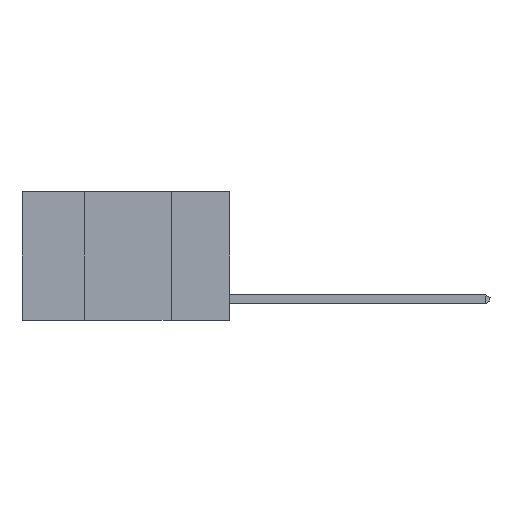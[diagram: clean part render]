
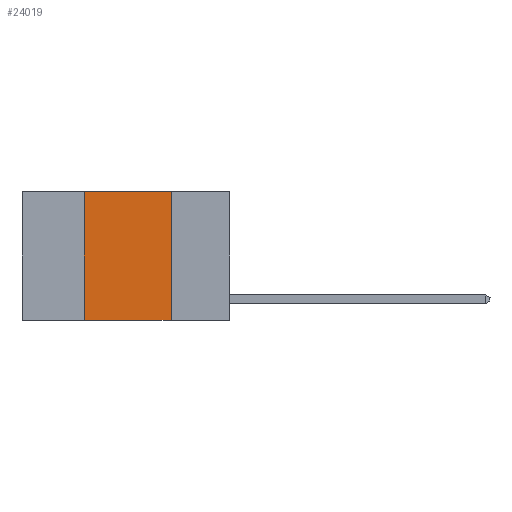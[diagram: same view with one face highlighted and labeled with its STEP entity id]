
A CAD part, left-side view. The second image highlights one B-rep face of the part: STEP entity #24019.
In plain terms, the highlighted planar face has unit normal (-1, 0, 0).
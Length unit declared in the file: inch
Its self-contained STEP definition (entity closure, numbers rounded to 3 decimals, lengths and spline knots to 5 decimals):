
#292 = LINE ( 'NONE', #28419, #7447 ) ;
#491 = CARTESIAN_POINT ( 'NONE',  ( 0., 0.17, 0. ) ) ;
#982 = EDGE_LOOP ( 'NONE', ( #23580, #26394, #14096, #22156 ) ) ;
#1614 = VECTOR ( 'NONE', #18758, 39.37008 ) ;
#3775 = EDGE_CURVE ( 'NONE', #6703, #23410, #18141, .T. ) ;
#4609 = CARTESIAN_POINT ( 'NONE',  ( 0., 0.6, -0.37 ) ) ;
#5477 = DIRECTION ( 'NONE',  ( 0., 0., -1. ) ) ;
#5719 = DIRECTION ( 'NONE',  ( 0., 0., -1. ) ) ;
#6703 = VERTEX_POINT ( 'NONE', #7699 ) ;
#6987 = DIRECTION ( 'NONE',  ( 0., 0., 1. ) ) ;
#7192 = LINE ( 'NONE', #4609, #1614 ) ;
#7447 = VECTOR ( 'NONE', #6987, 39.37008 ) ;
#7699 = CARTESIAN_POINT ( 'NONE',  ( 0., 0.42, 0. ) ) ;
#8982 = VECTOR ( 'NONE', #5719, 39.37008 ) ;
#11520 = VERTEX_POINT ( 'NONE', #12264 ) ;
#12264 = CARTESIAN_POINT ( 'NONE',  ( 0., 0.17, -0.37 ) ) ;
#12761 = CARTESIAN_POINT ( 'NONE',  ( 0., 0.6, 0. ) ) ;
#13286 = DIRECTION ( 'NONE',  ( 0., -1., 0. ) ) ;
#14096 = ORIENTED_EDGE ( 'NONE', *, *, #27547, .F. ) ;
#15358 = EDGE_CURVE ( 'NONE', #17722, #11520, #7192, .T. ) ;
#17275 = LINE ( 'NONE', #23964, #8982 ) ;
#17393 = VECTOR ( 'NONE', #13286, 39.37008 ) ;
#17722 = VERTEX_POINT ( 'NONE', #18951 ) ;
#18141 = LINE ( 'NONE', #29403, #17393 ) ;
#18758 = DIRECTION ( 'NONE',  ( 0., -1., 0. ) ) ;
#18951 = CARTESIAN_POINT ( 'NONE',  ( 0., 0.42, -0.37 ) ) ;
#19206 = EDGE_CURVE ( 'NONE', #23410, #11520, #17275, .T. ) ;
#22071 = DIRECTION ( 'NONE',  ( 1., 0., 0. ) ) ;
#22156 = ORIENTED_EDGE ( 'NONE', *, *, #15358, .T. ) ;
#23241 = AXIS2_PLACEMENT_3D ( 'NONE', #12761, #22071, #5477 ) ;
#23410 = VERTEX_POINT ( 'NONE', #491 ) ;
#23580 = ORIENTED_EDGE ( 'NONE', *, *, #19206, .F. ) ;
#23964 = CARTESIAN_POINT ( 'NONE',  ( 0., 0.17, 0. ) ) ;
#24019 = ADVANCED_FACE ( 'NONE', ( #28735 ), #26309, .F. ) ;
#26309 = PLANE ( 'NONE',  #23241 ) ;
#26394 = ORIENTED_EDGE ( 'NONE', *, *, #3775, .F. ) ;
#27547 = EDGE_CURVE ( 'NONE', #17722, #6703, #292, .T. ) ;
#28419 = CARTESIAN_POINT ( 'NONE',  ( 0., 0.42, 0. ) ) ;
#28735 = FACE_OUTER_BOUND ( 'NONE', #982, .T. ) ;
#29403 = CARTESIAN_POINT ( 'NONE',  ( 0., 0.6, 0. ) ) ;
